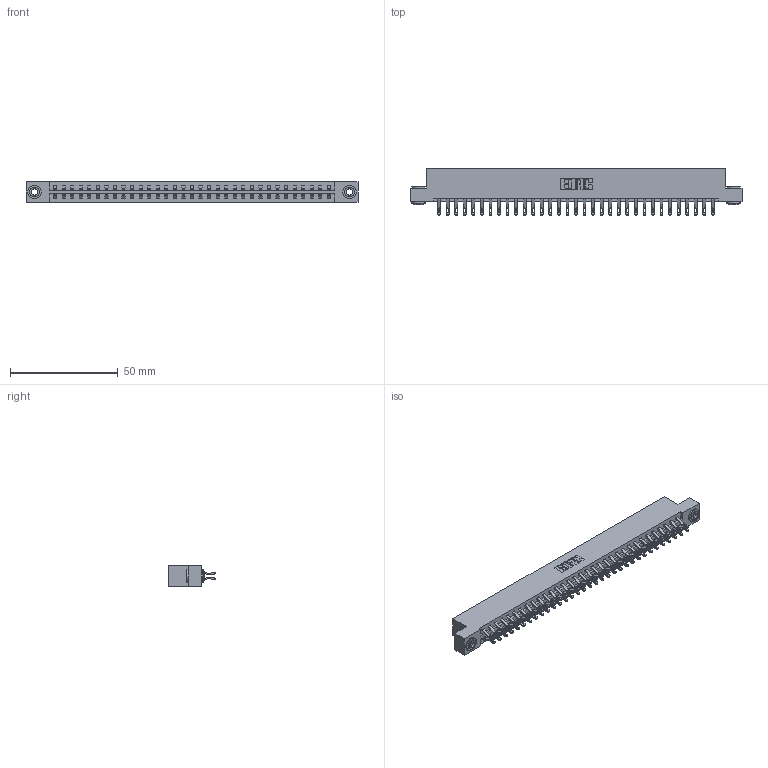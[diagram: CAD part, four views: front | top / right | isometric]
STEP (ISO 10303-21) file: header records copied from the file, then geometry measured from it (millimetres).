
FILE_DESCRIPTION (( 'STEP AP203' ), '1' );
FILE_NAME ('387-066-555-203.STEP', '2019-10-19T19:14:01', ( '' ), ( '' ), 'SwSTEP 2.0', 'SolidWorks 2016', '' );
FILE_SCHEMA (( 'CONFIG_CONTROL_DESIGN' ));
Length unit declared in the file: inch
Products named in the file (4): 337 Part_Flush Mounting Lugs - 0.156 Dia-TH; 345-250-002_345-250-002-102; 387-066-555-203; 345-292-001_555 Tail
Assembly tree (69 placements, depth 2):
  387-066-555-203
    337 Part_Flush Mounting Lugs - 0.156 Dia-TH
    345-292-001_555 Tail  x66
    345-250-002_345-250-002-102  x2
Bounding box: 153.77 x 21.47 x 9.4 mm (x, y, z)
Volume: 16296.7 mm3; surface area: 19281.9 mm2
Topology: 69 solids, 69 shells, 4112 faces, 12861 edges, 8570 vertices
Faces by surface type: plane 2456, cylinder 1648, cone 8
Entity records: 27726 total; most frequent: CARTESIAN_POINT 4687, ORIENTED_EDGE 4586, DIRECTION 4007, EDGE_CURVE 2293, LINE 2121, VECTOR 2121, VERTEX_POINT 1526, AXIS2_PLACEMENT_3D 943
